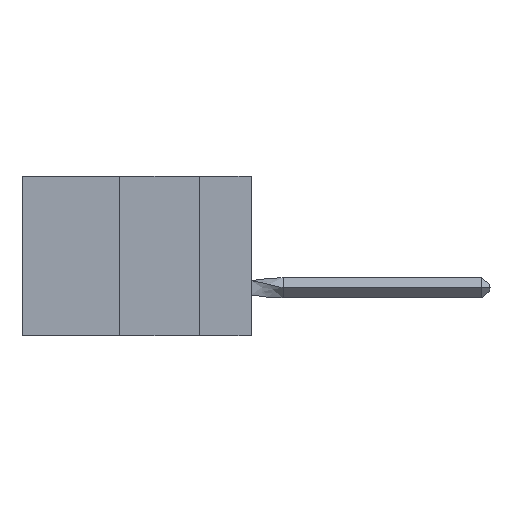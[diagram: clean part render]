
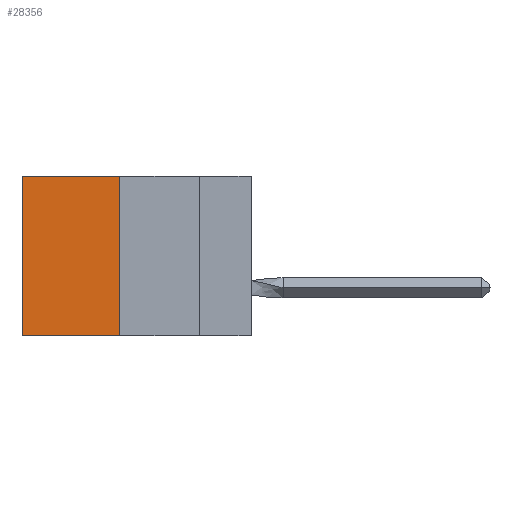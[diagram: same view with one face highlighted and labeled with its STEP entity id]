
A CAD part, left-side view. The second image highlights one B-rep face of the part: STEP entity #28356.
In plain terms, the highlighted planar face has unit normal (-1, 0, 0).
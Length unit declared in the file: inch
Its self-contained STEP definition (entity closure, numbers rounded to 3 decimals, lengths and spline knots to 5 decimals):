
#76 = VERTEX_POINT ( 'NONE', #33480 ) ;
#145 = ORIENTED_EDGE ( 'NONE', *, *, #11315, .F. ) ;
#741 = DIRECTION ( 'NONE',  ( 0., 0., -1. ) ) ;
#1765 = ORIENTED_EDGE ( 'NONE', *, *, #19738, .F. ) ;
#2239 = FACE_OUTER_BOUND ( 'NONE', #24750, .T. ) ;
#4432 = VECTOR ( 'NONE', #741, 39.37008 ) ;
#4631 = CARTESIAN_POINT ( 'NONE',  ( 0.305, 0.72, 0. ) ) ;
#6097 = VERTEX_POINT ( 'NONE', #8601 ) ;
#8601 = CARTESIAN_POINT ( 'NONE',  ( 0.305, 0.413, 0. ) ) ;
#9977 = DIRECTION ( 'NONE',  ( 0., 1., 0. ) ) ;
#10246 = EDGE_CURVE ( 'NONE', #6097, #12434, #36404, .T. ) ;
#10871 = LINE ( 'NONE', #30105, #4432 ) ;
#11315 = EDGE_CURVE ( 'NONE', #6097, #14937, #10871, .T. ) ;
#12058 = DIRECTION ( 'NONE',  ( 0., 0., -1. ) ) ;
#12434 = VERTEX_POINT ( 'NONE', #4631 ) ;
#14130 = AXIS2_PLACEMENT_3D ( 'NONE', #23504, #35412, #12058 ) ;
#14138 = DIRECTION ( 'NONE',  ( 0., 1., 0. ) ) ;
#14937 = VERTEX_POINT ( 'NONE', #26064 ) ;
#14959 = PLANE ( 'NONE',  #14130 ) ;
#18341 = VECTOR ( 'NONE', #37103, 39.37008 ) ;
#19738 = EDGE_CURVE ( 'NONE', #14937, #76, #35278, .T. ) ;
#19967 = CARTESIAN_POINT ( 'NONE',  ( 0.305, 0.413, 0. ) ) ;
#22050 = CARTESIAN_POINT ( 'NONE',  ( 0.305, 0.413, -0.5 ) ) ;
#22195 = VECTOR ( 'NONE', #14138, 39.37008 ) ;
#23504 = CARTESIAN_POINT ( 'NONE',  ( 0.305, 0.413, -0.5 ) ) ;
#24304 = VECTOR ( 'NONE', #9977, 39.37008 ) ;
#24750 = EDGE_LOOP ( 'NONE', ( #35592, #1765, #145, #26943 ) ) ;
#26064 = CARTESIAN_POINT ( 'NONE',  ( 0.305, 0.413, -0.5 ) ) ;
#26558 = EDGE_CURVE ( 'NONE', #12434, #76, #30698, .T. ) ;
#26943 = ORIENTED_EDGE ( 'NONE', *, *, #10246, .T. ) ;
#28356 = ADVANCED_FACE ( 'NONE', ( #2239 ), #14959, .F. ) ;
#30105 = CARTESIAN_POINT ( 'NONE',  ( 0.305, 0.413, -0.5 ) ) ;
#30698 = LINE ( 'NONE', #33911, #18341 ) ;
#33480 = CARTESIAN_POINT ( 'NONE',  ( 0.305, 0.72, -0.5 ) ) ;
#33911 = CARTESIAN_POINT ( 'NONE',  ( 0.305, 0.72, -0.5 ) ) ;
#35278 = LINE ( 'NONE', #22050, #24304 ) ;
#35412 = DIRECTION ( 'NONE',  ( 1., 0., 0. ) ) ;
#35592 = ORIENTED_EDGE ( 'NONE', *, *, #26558, .T. ) ;
#36404 = LINE ( 'NONE', #19967, #22195 ) ;
#37103 = DIRECTION ( 'NONE',  ( 0., 0., -1. ) ) ;
